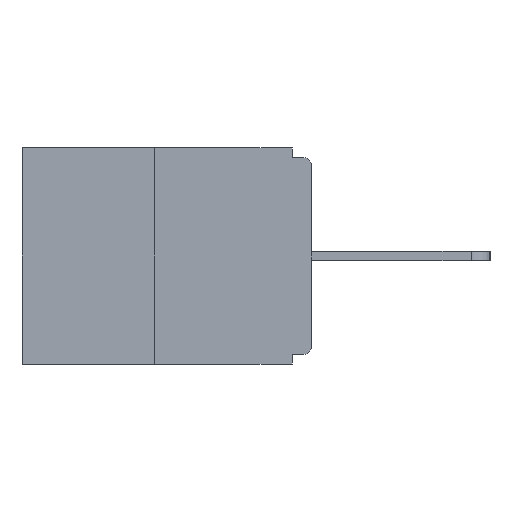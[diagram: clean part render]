
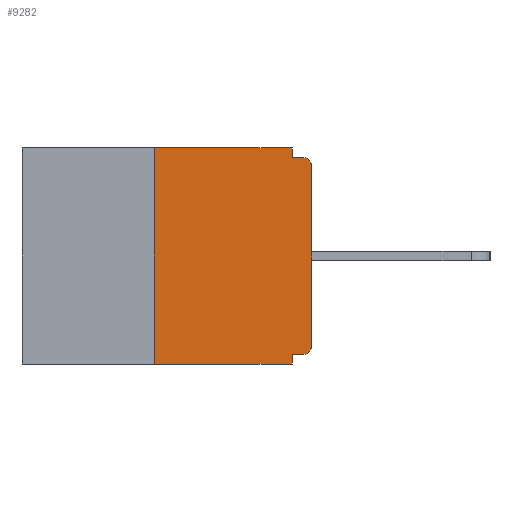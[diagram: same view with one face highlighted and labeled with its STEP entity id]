
A CAD part, left-side view. The second image highlights one B-rep face of the part: STEP entity #9282.
In plain terms, the highlighted planar face has unit normal (-1, 0, 0).
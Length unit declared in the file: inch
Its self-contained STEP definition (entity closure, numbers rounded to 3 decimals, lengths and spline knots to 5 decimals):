
#177 = LINE ( 'NONE', #15929, #7636 ) ;
#208 = AXIS2_PLACEMENT_3D ( 'NONE', #15684, #17139, #8145 ) ;
#493 = ORIENTED_EDGE ( 'NONE', *, *, #8773, .F. ) ;
#497 = LINE ( 'NONE', #15810, #17781 ) ;
#509 = EDGE_CURVE ( 'NONE', #17277, #1456, #497, .T. ) ;
#715 = DIRECTION ( 'NONE',  ( 0., 0., -1. ) ) ;
#1456 = VERTEX_POINT ( 'NONE', #11207 ) ;
#1577 = CARTESIAN_POINT ( 'NONE',  ( 0., 0.25, -0.343 ) ) ;
#1938 = EDGE_CURVE ( 'NONE', #13510, #12468, #16371, .T. ) ;
#2081 = EDGE_CURVE ( 'NONE', #5508, #2538, #17946, .T. ) ;
#2249 = CARTESIAN_POINT ( 'NONE',  ( 0., 0.015, -0.313 ) ) ;
#2444 = CARTESIAN_POINT ( 'NONE',  ( 0., 0.031, -0.343 ) ) ;
#2538 = VERTEX_POINT ( 'NONE', #9656 ) ;
#2602 = DIRECTION ( 'NONE',  ( -1., 0., 0. ) ) ;
#2666 = DIRECTION ( 'NONE',  ( 0., -1., 0. ) ) ;
#3468 = CARTESIAN_POINT ( 'NONE',  ( 0., 0.015, -0.328 ) ) ;
#3497 = CARTESIAN_POINT ( 'NONE',  ( 0., 0.46, 0. ) ) ;
#3506 = ORIENTED_EDGE ( 'NONE', *, *, #6300, .T. ) ;
#3850 = DIRECTION ( 'NONE',  ( 0., 0., -1. ) ) ;
#4029 = VERTEX_POINT ( 'NONE', #18218 ) ;
#4212 = DIRECTION ( 'NONE',  ( 0., -1., 0. ) ) ;
#4476 = CIRCLE ( 'NONE', #16269, 0.015 ) ;
#4838 = CIRCLE ( 'NONE', #8986, 0.015 ) ;
#5000 = PLANE ( 'NONE',  #208 ) ;
#5069 = DIRECTION ( 'NONE',  ( 0., -1., 0. ) ) ;
#5508 = VERTEX_POINT ( 'NONE', #3468 ) ;
#5717 = LINE ( 'NONE', #2444, #16879 ) ;
#5769 = CARTESIAN_POINT ( 'NONE',  ( 0., 0.031, -0.343 ) ) ;
#6300 = EDGE_CURVE ( 'NONE', #18600, #10016, #177, .T. ) ;
#6918 = CARTESIAN_POINT ( 'NONE',  ( 0., 0.031, 0. ) ) ;
#6932 = ORIENTED_EDGE ( 'NONE', *, *, #509, .T. ) ;
#7186 = ORIENTED_EDGE ( 'NONE', *, *, #13300, .F. ) ;
#7636 = VECTOR ( 'NONE', #2666, 39.37008 ) ;
#8145 = DIRECTION ( 'NONE',  ( 0., 0., -1. ) ) ;
#8166 = ORIENTED_EDGE ( 'NONE', *, *, #11225, .F. ) ;
#8497 = LINE ( 'NONE', #16865, #16036 ) ;
#8504 = EDGE_CURVE ( 'NONE', #18600, #4029, #8497, .T. ) ;
#8773 = EDGE_CURVE ( 'NONE', #11775, #13510, #14943, .T. ) ;
#8809 = EDGE_LOOP ( 'NONE', ( #7186, #15294, #3506, #8166, #13765, #10102, #6932, #12111, #12599, #493 ) ) ;
#8986 = AXIS2_PLACEMENT_3D ( 'NONE', #11999, #2602, #13531 ) ;
#9282 = ADVANCED_FACE ( 'NONE', ( #16707 ), #5000, .F. ) ;
#9656 = CARTESIAN_POINT ( 'NONE',  ( 0., 0.031, -0.328 ) ) ;
#9836 = VECTOR ( 'NONE', #10828, 39.37008 ) ;
#10016 = VERTEX_POINT ( 'NONE', #5769 ) ;
#10102 = ORIENTED_EDGE ( 'NONE', *, *, #15137, .T. ) ;
#10611 = CARTESIAN_POINT ( 'NONE',  ( 0., 0., -0.015 ) ) ;
#10828 = DIRECTION ( 'NONE',  ( 0., 1., 0. ) ) ;
#11207 = CARTESIAN_POINT ( 'NONE',  ( 0., 0., -0.03 ) ) ;
#11225 = EDGE_CURVE ( 'NONE', #2538, #10016, #5717, .T. ) ;
#11579 = DIRECTION ( 'NONE',  ( 0., 0., -1. ) ) ;
#11775 = VERTEX_POINT ( 'NONE', #13489 ) ;
#11999 = CARTESIAN_POINT ( 'NONE',  ( 0., 0.015, -0.03 ) ) ;
#12111 = ORIENTED_EDGE ( 'NONE', *, *, #12451, .T. ) ;
#12451 = EDGE_CURVE ( 'NONE', #1456, #12468, #4838, .T. ) ;
#12468 = VERTEX_POINT ( 'NONE', #17770 ) ;
#12517 = DIRECTION ( 'NONE',  ( 0., 0., 1. ) ) ;
#12599 = ORIENTED_EDGE ( 'NONE', *, *, #1938, .F. ) ;
#13092 = CARTESIAN_POINT ( 'NONE',  ( 0., 0., -0.313 ) ) ;
#13107 = VECTOR ( 'NONE', #5069, 39.37008 ) ;
#13207 = DIRECTION ( 'NONE',  ( -1., 0., 0. ) ) ;
#13300 = EDGE_CURVE ( 'NONE', #4029, #11775, #13580, .T. ) ;
#13489 = CARTESIAN_POINT ( 'NONE',  ( 0., 0.031, 0. ) ) ;
#13510 = VERTEX_POINT ( 'NONE', #14900 ) ;
#13531 = DIRECTION ( 'NONE',  ( 0., 0., -1. ) ) ;
#13580 = LINE ( 'NONE', #3497, #13107 ) ;
#13765 = ORIENTED_EDGE ( 'NONE', *, *, #2081, .F. ) ;
#14900 = CARTESIAN_POINT ( 'NONE',  ( 0., 0.031, -0.015 ) ) ;
#14943 = LINE ( 'NONE', #6918, #18268 ) ;
#15137 = EDGE_CURVE ( 'NONE', #5508, #17277, #4476, .T. ) ;
#15294 = ORIENTED_EDGE ( 'NONE', *, *, #8504, .F. ) ;
#15684 = CARTESIAN_POINT ( 'NONE',  ( 0., 0.46, 0. ) ) ;
#15810 = CARTESIAN_POINT ( 'NONE',  ( 0., 0., 0. ) ) ;
#15929 = CARTESIAN_POINT ( 'NONE',  ( 0., 0.46, -0.343 ) ) ;
#15996 = CARTESIAN_POINT ( 'NONE',  ( 0., 0., -0.328 ) ) ;
#16036 = VECTOR ( 'NONE', #12517, 39.37008 ) ;
#16269 = AXIS2_PLACEMENT_3D ( 'NONE', #2249, #13207, #3850 ) ;
#16371 = LINE ( 'NONE', #10611, #19668 ) ;
#16450 = DIRECTION ( 'NONE',  ( 0., 0., 1. ) ) ;
#16707 = FACE_OUTER_BOUND ( 'NONE', #8809, .T. ) ;
#16865 = CARTESIAN_POINT ( 'NONE',  ( 0., 0.25, 0. ) ) ;
#16879 = VECTOR ( 'NONE', #715, 39.37008 ) ;
#17139 = DIRECTION ( 'NONE',  ( 1., 0., 0. ) ) ;
#17277 = VERTEX_POINT ( 'NONE', #13092 ) ;
#17770 = CARTESIAN_POINT ( 'NONE',  ( 0., 0.015, -0.015 ) ) ;
#17781 = VECTOR ( 'NONE', #16450, 39.37008 ) ;
#17946 = LINE ( 'NONE', #15996, #9836 ) ;
#18218 = CARTESIAN_POINT ( 'NONE',  ( 0., 0.25, 0. ) ) ;
#18268 = VECTOR ( 'NONE', #11579, 39.37008 ) ;
#18600 = VERTEX_POINT ( 'NONE', #1577 ) ;
#19668 = VECTOR ( 'NONE', #4212, 39.37008 ) ;
